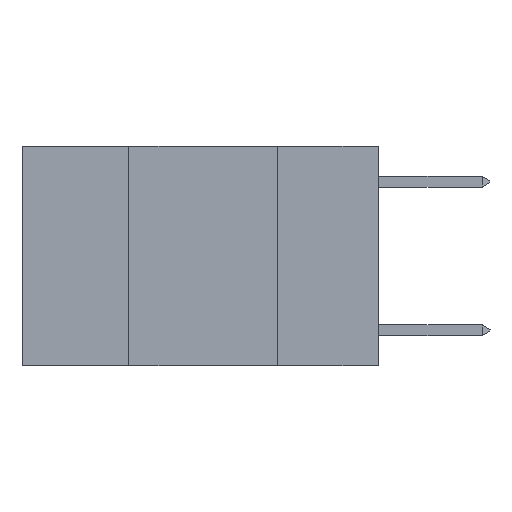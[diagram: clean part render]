
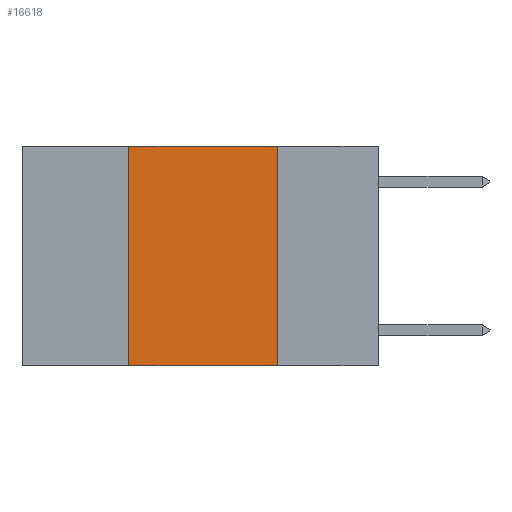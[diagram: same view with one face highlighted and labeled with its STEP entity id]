
A CAD part, left-side view. The second image highlights one B-rep face of the part: STEP entity #16618.
In plain terms, the highlighted planar face has unit normal (-1, 0, 0).
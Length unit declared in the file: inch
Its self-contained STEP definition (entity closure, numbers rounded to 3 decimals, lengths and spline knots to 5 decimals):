
#161 = ORIENTED_EDGE ( 'NONE', *, *, #2590, .F. ) ;
#1779 = EDGE_CURVE ( 'NONE', #20733, #17677, #5685, .T. ) ;
#1862 = LINE ( 'NONE', #4369, #1903 ) ;
#1903 = VECTOR ( 'NONE', #9291, 39.37008 ) ;
#2238 = VERTEX_POINT ( 'NONE', #8615 ) ;
#2536 = CARTESIAN_POINT ( 'NONE',  ( 0., 0.17, 0. ) ) ;
#2590 = EDGE_CURVE ( 'NONE', #2238, #20733, #1862, .T. ) ;
#4132 = CARTESIAN_POINT ( 'NONE',  ( 0., 0.17, 0. ) ) ;
#4369 = CARTESIAN_POINT ( 'NONE',  ( 0., 0.42, 0. ) ) ;
#5655 = FACE_OUTER_BOUND ( 'NONE', #18885, .T. ) ;
#5660 = PLANE ( 'NONE',  #14179 ) ;
#5661 = VECTOR ( 'NONE', #15744, 39.37008 ) ;
#5685 = LINE ( 'NONE', #19114, #5661 ) ;
#7348 = CARTESIAN_POINT ( 'NONE',  ( 0., 0.6, -0.37 ) ) ;
#7680 = DIRECTION ( 'NONE',  ( 0., 0., -1. ) ) ;
#7792 = VECTOR ( 'NONE', #7680, 39.37008 ) ;
#7879 = LINE ( 'NONE', #4132, #7792 ) ;
#7950 = EDGE_CURVE ( 'NONE', #17677, #17297, #7879, .T. ) ;
#8615 = CARTESIAN_POINT ( 'NONE',  ( 0., 0.42, -0.37 ) ) ;
#9107 = DIRECTION ( 'NONE',  ( 1., 0., 0. ) ) ;
#9189 = EDGE_CURVE ( 'NONE', #2238, #17297, #15435, .T. ) ;
#9291 = DIRECTION ( 'NONE',  ( 0., 0., 1. ) ) ;
#10134 = ORIENTED_EDGE ( 'NONE', *, *, #7950, .F. ) ;
#13735 = ORIENTED_EDGE ( 'NONE', *, *, #1779, .F. ) ;
#14179 = AXIS2_PLACEMENT_3D ( 'NONE', #18969, #9107, #20444 ) ;
#14620 = ORIENTED_EDGE ( 'NONE', *, *, #9189, .T. ) ;
#15182 = CARTESIAN_POINT ( 'NONE',  ( 0., 0.17, -0.37 ) ) ;
#15435 = LINE ( 'NONE', #7348, #15492 ) ;
#15492 = VECTOR ( 'NONE', #18964, 39.37008 ) ;
#15744 = DIRECTION ( 'NONE',  ( 0., -1., 0. ) ) ;
#16618 = ADVANCED_FACE ( 'NONE', ( #5655 ), #5660, .F. ) ;
#17297 = VERTEX_POINT ( 'NONE', #15182 ) ;
#17677 = VERTEX_POINT ( 'NONE', #2536 ) ;
#18885 = EDGE_LOOP ( 'NONE', ( #10134, #13735, #161, #14620 ) ) ;
#18964 = DIRECTION ( 'NONE',  ( 0., -1., 0. ) ) ;
#18969 = CARTESIAN_POINT ( 'NONE',  ( 0., 0.6, 0. ) ) ;
#19114 = CARTESIAN_POINT ( 'NONE',  ( 0., 0.6, 0. ) ) ;
#20444 = DIRECTION ( 'NONE',  ( 0., 0., -1. ) ) ;
#20733 = VERTEX_POINT ( 'NONE', #20830 ) ;
#20830 = CARTESIAN_POINT ( 'NONE',  ( 0., 0.42, 0. ) ) ;
